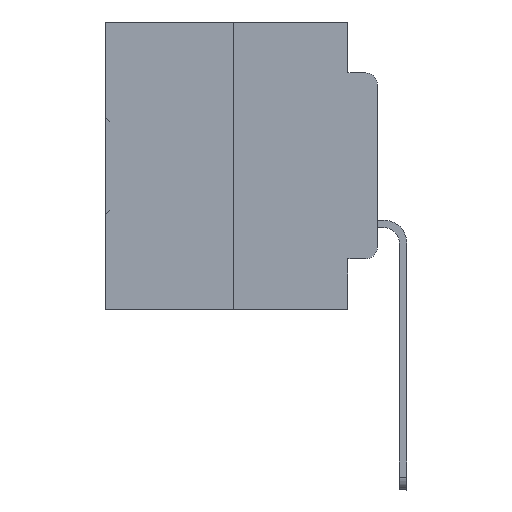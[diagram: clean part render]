
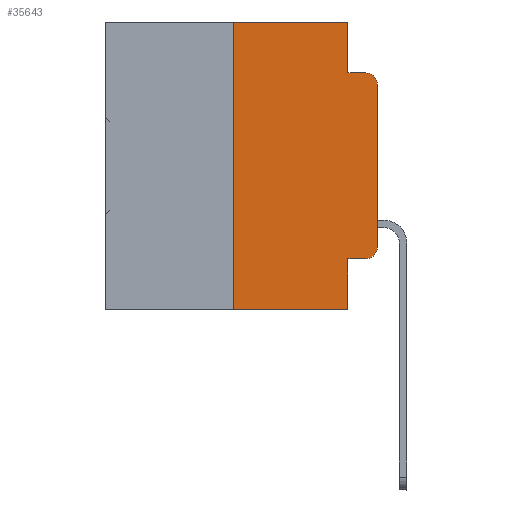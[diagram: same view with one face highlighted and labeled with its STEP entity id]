
A CAD part, left-side view. The second image highlights one B-rep face of the part: STEP entity #35643.
In plain terms, the highlighted planar face has unit normal (-1, 0, 0).
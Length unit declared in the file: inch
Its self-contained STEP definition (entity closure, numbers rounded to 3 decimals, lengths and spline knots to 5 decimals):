
#320 = LINE ( 'NONE', #2494, #4218 ) ;
#500 = VECTOR ( 'NONE', #34777, 39.37008 ) ;
#651 = VERTEX_POINT ( 'NONE', #8683 ) ;
#762 = DIRECTION ( 'NONE',  ( -1., 0., 0. ) ) ;
#1421 = VERTEX_POINT ( 'NONE', #13294 ) ;
#1681 = CARTESIAN_POINT ( 'NONE',  ( 0., 0.051, -0.4115 ) ) ;
#1908 = VERTEX_POINT ( 'NONE', #30458 ) ;
#1976 = CARTESIAN_POINT ( 'NONE',  ( 0., 0.051, 0. ) ) ;
#2338 = DIRECTION ( 'NONE',  ( 1., 0., 0. ) ) ;
#2376 = CARTESIAN_POINT ( 'NONE',  ( 0., 0., -0.1085 ) ) ;
#2393 = LINE ( 'NONE', #32862, #26994 ) ;
#2494 = CARTESIAN_POINT ( 'NONE',  ( 0., 0.473, -0.5 ) ) ;
#4203 = VERTEX_POINT ( 'NONE', #30040 ) ;
#4218 = VECTOR ( 'NONE', #14103, 39.37008 ) ;
#4358 = LINE ( 'NONE', #29201, #5968 ) ;
#4500 = CIRCLE ( 'NONE', #35198, 0.02 ) ;
#4648 = CIRCLE ( 'NONE', #7532, 0.02 ) ;
#4742 = DIRECTION ( 'NONE',  ( -1., 0., 0. ) ) ;
#4863 = ORIENTED_EDGE ( 'NONE', *, *, #35490, .F. ) ;
#5069 = FACE_OUTER_BOUND ( 'NONE', #9922, .T. ) ;
#5607 = CARTESIAN_POINT ( 'NONE',  ( 0., 0.25, 0. ) ) ;
#5968 = VECTOR ( 'NONE', #18665, 39.37008 ) ;
#6120 = CARTESIAN_POINT ( 'NONE',  ( 0., 0.02, -0.0885 ) ) ;
#6765 = DIRECTION ( 'NONE',  ( 0., -1., 0. ) ) ;
#6895 = LINE ( 'NONE', #21037, #7387 ) ;
#6932 = CARTESIAN_POINT ( 'NONE',  ( 0., 0.02, -0.3915 ) ) ;
#7050 = EDGE_CURVE ( 'NONE', #22819, #1421, #2393, .T. ) ;
#7289 = DIRECTION ( 'NONE',  ( 0., 0., 1. ) ) ;
#7387 = VECTOR ( 'NONE', #26290, 39.37008 ) ;
#7532 = AXIS2_PLACEMENT_3D ( 'NONE', #16913, #762, #14549 ) ;
#8657 = EDGE_CURVE ( 'NONE', #1908, #30438, #32116, .T. ) ;
#8683 = CARTESIAN_POINT ( 'NONE',  ( 0., 0.25, -0.5 ) ) ;
#9501 = VERTEX_POINT ( 'NONE', #19451 ) ;
#9578 = LINE ( 'NONE', #34950, #500 ) ;
#9922 = EDGE_LOOP ( 'NONE', ( #22268, #12099, #4863, #14932, #12831, #17772, #25202, #21925, #30619, #12112 ) ) ;
#12099 = ORIENTED_EDGE ( 'NONE', *, *, #16927, .T. ) ;
#12112 = ORIENTED_EDGE ( 'NONE', *, *, #12729, .T. ) ;
#12211 = VERTEX_POINT ( 'NONE', #6120 ) ;
#12729 = EDGE_CURVE ( 'NONE', #9501, #1908, #4500, .T. ) ;
#12831 = ORIENTED_EDGE ( 'NONE', *, *, #7050, .F. ) ;
#13052 = DIRECTION ( 'NONE',  ( 0., 0., -1. ) ) ;
#13294 = CARTESIAN_POINT ( 'NONE',  ( 0., 0.051, 0. ) ) ;
#13502 = AXIS2_PLACEMENT_3D ( 'NONE', #30618, #2338, #35523 ) ;
#14103 = DIRECTION ( 'NONE',  ( 0., -1., 0. ) ) ;
#14549 = DIRECTION ( 'NONE',  ( 0., 0., -1. ) ) ;
#14932 = ORIENTED_EDGE ( 'NONE', *, *, #21549, .F. ) ;
#15254 = CARTESIAN_POINT ( 'NONE',  ( 0., 0., 0. ) ) ;
#15633 = DIRECTION ( 'NONE',  ( 0., 0., -1. ) ) ;
#16130 = PLANE ( 'NONE',  #13502 ) ;
#16721 = VECTOR ( 'NONE', #6765, 39.37008 ) ;
#16913 = CARTESIAN_POINT ( 'NONE',  ( 0., 0.02, -0.1085 ) ) ;
#16927 = EDGE_CURVE ( 'NONE', #30438, #12211, #4648, .T. ) ;
#17396 = VERTEX_POINT ( 'NONE', #22490 ) ;
#17573 = VECTOR ( 'NONE', #7289, 39.37008 ) ;
#17772 = ORIENTED_EDGE ( 'NONE', *, *, #29055, .F. ) ;
#18162 = CARTESIAN_POINT ( 'NONE',  ( 0., 0.051, -0.4115 ) ) ;
#18665 = DIRECTION ( 'NONE',  ( 0., -1., 0. ) ) ;
#19451 = CARTESIAN_POINT ( 'NONE',  ( 0., 0.02, -0.4115 ) ) ;
#19813 = VERTEX_POINT ( 'NONE', #18162 ) ;
#21037 = CARTESIAN_POINT ( 'NONE',  ( 0., 0.25, 0. ) ) ;
#21549 = EDGE_CURVE ( 'NONE', #1421, #17396, #21561, .T. ) ;
#21561 = LINE ( 'NONE', #1976, #30817 ) ;
#21697 = EDGE_CURVE ( 'NONE', #651, #4203, #320, .T. ) ;
#21925 = ORIENTED_EDGE ( 'NONE', *, *, #30757, .F. ) ;
#22268 = ORIENTED_EDGE ( 'NONE', *, *, #8657, .T. ) ;
#22490 = CARTESIAN_POINT ( 'NONE',  ( 0., 0.051, -0.0885 ) ) ;
#22819 = VERTEX_POINT ( 'NONE', #5607 ) ;
#25202 = ORIENTED_EDGE ( 'NONE', *, *, #21697, .T. ) ;
#26290 = DIRECTION ( 'NONE',  ( 0., 0., 1. ) ) ;
#26994 = VECTOR ( 'NONE', #32674, 39.37008 ) ;
#29055 = EDGE_CURVE ( 'NONE', #651, #22819, #6895, .T. ) ;
#29201 = CARTESIAN_POINT ( 'NONE',  ( 0., 0.051, -0.0885 ) ) ;
#30040 = CARTESIAN_POINT ( 'NONE',  ( 0., 0.051, -0.5 ) ) ;
#30301 = EDGE_CURVE ( 'NONE', #19813, #9501, #32140, .T. ) ;
#30438 = VERTEX_POINT ( 'NONE', #2376 ) ;
#30458 = CARTESIAN_POINT ( 'NONE',  ( 0., 0., -0.3915 ) ) ;
#30618 = CARTESIAN_POINT ( 'NONE',  ( 0., 0.473, 0. ) ) ;
#30619 = ORIENTED_EDGE ( 'NONE', *, *, #30301, .T. ) ;
#30757 = EDGE_CURVE ( 'NONE', #19813, #4203, #9578, .T. ) ;
#30817 = VECTOR ( 'NONE', #13052, 39.37008 ) ;
#32116 = LINE ( 'NONE', #15254, #17573 ) ;
#32140 = LINE ( 'NONE', #1681, #16721 ) ;
#32674 = DIRECTION ( 'NONE',  ( 0., -1., 0. ) ) ;
#32862 = CARTESIAN_POINT ( 'NONE',  ( 0., 0.473, 0. ) ) ;
#34777 = DIRECTION ( 'NONE',  ( 0., 0., -1. ) ) ;
#34950 = CARTESIAN_POINT ( 'NONE',  ( 0., 0.051, 0. ) ) ;
#35198 = AXIS2_PLACEMENT_3D ( 'NONE', #6932, #4742, #15633 ) ;
#35490 = EDGE_CURVE ( 'NONE', #17396, #12211, #4358, .T. ) ;
#35523 = DIRECTION ( 'NONE',  ( 0., 0., -1. ) ) ;
#35643 = ADVANCED_FACE ( 'NONE', ( #5069 ), #16130, .F. ) ;
